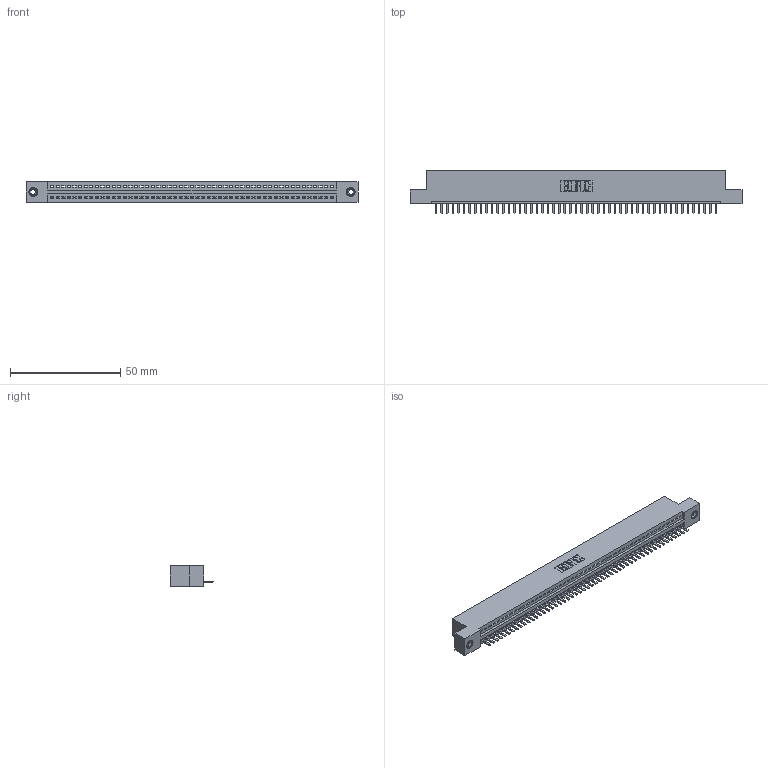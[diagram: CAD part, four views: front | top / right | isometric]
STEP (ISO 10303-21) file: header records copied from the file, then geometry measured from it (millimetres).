
FILE_DESCRIPTION (( 'STEP AP203' ), '1' );
FILE_NAME ('345-051-520-108.STEP', '2018-09-22T16:23:33', ( '' ), ( '' ), 'SwSTEP 2.0', 'SolidWorks 2016', '' );
FILE_SCHEMA (( 'CONFIG_CONTROL_DESIGN' ));
Length unit declared in the file: inch
Products named in the file (4): 345 Part_Flush Mounting Lugs - 0.156 Dia-TI; 345-292-001_345-293-120; 345-250-001_345-250-003-102; 345-051-520-108
Assembly tree (54 placements, depth 2):
  345-051-520-108
    345 Part_Flush Mounting Lugs - 0.156 Dia-TI
    345-292-001_345-293-120  x51
    345-250-001_345-250-003-102  x2
Bounding box: 150.75 x 19.68 x 9.4 mm (x, y, z)
Volume: 14238.8 mm3; surface area: 18583.6 mm2
Topology: 54 solids, 54 shells, 3348 faces, 9861 edges, 6430 vertices
Faces by surface type: plane 2254, cylinder 1078, cone 12, torus 4
Entity records: 38472 total; most frequent: CARTESIAN_POINT 6656, ORIENTED_EDGE 6622, DIRECTION 5815, EDGE_CURVE 3311, VECTOR 2951, LINE 2951, VERTEX_POINT 2200, AXIS2_PLACEMENT_3D 1432
